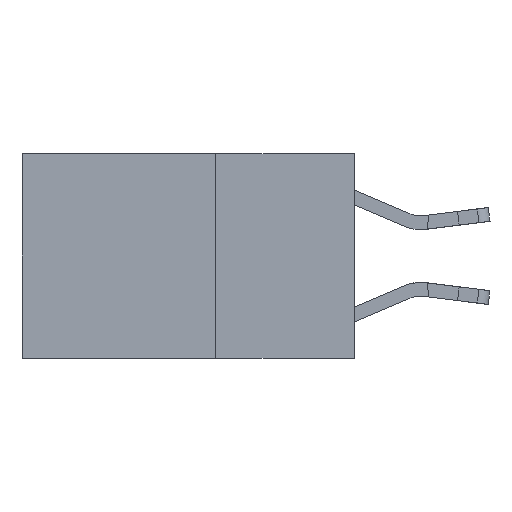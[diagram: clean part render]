
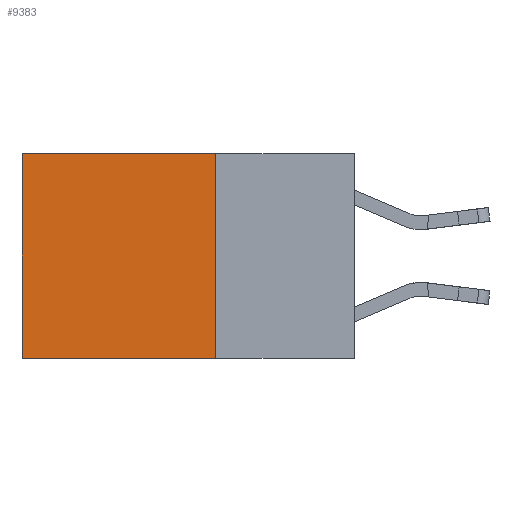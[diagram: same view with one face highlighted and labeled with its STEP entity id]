
A CAD part, left-side view. The second image highlights one B-rep face of the part: STEP entity #9383.
In plain terms, the highlighted planar face has unit normal (-1, 0, 0).
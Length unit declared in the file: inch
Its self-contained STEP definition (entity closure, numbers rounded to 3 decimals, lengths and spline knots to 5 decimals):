
#1306 = DIRECTION ( 'NONE',  ( 0., 1., 0. ) ) ;
#1465 = LINE ( 'NONE', #8646, #8526 ) ;
#1910 = DIRECTION ( 'NONE',  ( 0., 0., -1. ) ) ;
#2970 = CARTESIAN_POINT ( 'NONE',  ( 0.2625, 0.25, 0. ) ) ;
#3873 = ORIENTED_EDGE ( 'NONE', *, *, #17524, .F. ) ;
#4343 = VECTOR ( 'NONE', #1910, 39.37008 ) ;
#5666 = FACE_OUTER_BOUND ( 'NONE', #6328, .T. ) ;
#6316 = CARTESIAN_POINT ( 'NONE',  ( 0.2625, 0.25, -0.37 ) ) ;
#6328 = EDGE_LOOP ( 'NONE', ( #13377, #3873, #10870, #8695 ) ) ;
#7503 = LINE ( 'NONE', #11717, #4343 ) ;
#7637 = AXIS2_PLACEMENT_3D ( 'NONE', #2970, #10057, #15572 ) ;
#7973 = VECTOR ( 'NONE', #1306, 39.37008 ) ;
#8392 = LINE ( 'NONE', #11204, #7973 ) ;
#8526 = VECTOR ( 'NONE', #14349, 39.37008 ) ;
#8646 = CARTESIAN_POINT ( 'NONE',  ( 0.2625, 0.6, 0. ) ) ;
#8695 = ORIENTED_EDGE ( 'NONE', *, *, #16536, .T. ) ;
#9383 = ADVANCED_FACE ( 'NONE', ( #5666 ), #11342, .F. ) ;
#9699 = LINE ( 'NONE', #12866, #11546 ) ;
#10057 = DIRECTION ( 'NONE',  ( 1., 0., 0. ) ) ;
#10759 = EDGE_CURVE ( 'NONE', #14770, #13189, #1465, .T. ) ;
#10870 = ORIENTED_EDGE ( 'NONE', *, *, #14442, .F. ) ;
#11204 = CARTESIAN_POINT ( 'NONE',  ( 0.2625, 0.25, -0.37 ) ) ;
#11342 = PLANE ( 'NONE',  #7637 ) ;
#11546 = VECTOR ( 'NONE', #15410, 39.37008 ) ;
#11717 = CARTESIAN_POINT ( 'NONE',  ( 0.2625, 0.25, 0. ) ) ;
#12866 = CARTESIAN_POINT ( 'NONE',  ( 0.2625, 0.25, 0. ) ) ;
#12898 = VERTEX_POINT ( 'NONE', #6316 ) ;
#13189 = VERTEX_POINT ( 'NONE', #17337 ) ;
#13377 = ORIENTED_EDGE ( 'NONE', *, *, #10759, .T. ) ;
#14349 = DIRECTION ( 'NONE',  ( 0., 0., -1. ) ) ;
#14442 = EDGE_CURVE ( 'NONE', #17488, #12898, #7503, .T. ) ;
#14770 = VERTEX_POINT ( 'NONE', #18437 ) ;
#15410 = DIRECTION ( 'NONE',  ( 0., 1., 0. ) ) ;
#15572 = DIRECTION ( 'NONE',  ( 0., 0., -1. ) ) ;
#15881 = CARTESIAN_POINT ( 'NONE',  ( 0.2625, 0.25, 0. ) ) ;
#16536 = EDGE_CURVE ( 'NONE', #17488, #14770, #9699, .T. ) ;
#17337 = CARTESIAN_POINT ( 'NONE',  ( 0.2625, 0.6, -0.37 ) ) ;
#17488 = VERTEX_POINT ( 'NONE', #15881 ) ;
#17524 = EDGE_CURVE ( 'NONE', #12898, #13189, #8392, .T. ) ;
#18437 = CARTESIAN_POINT ( 'NONE',  ( 0.2625, 0.6, 0. ) ) ;
